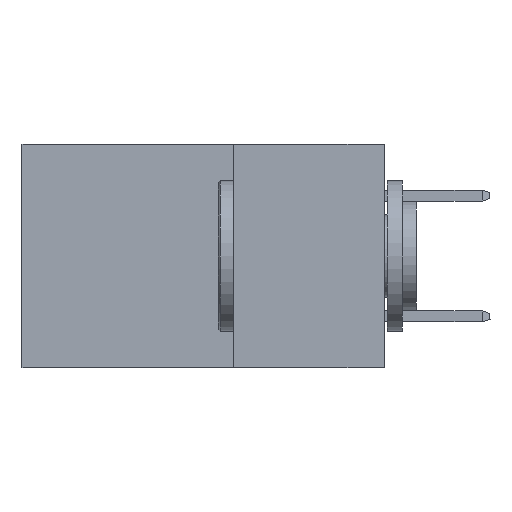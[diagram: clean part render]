
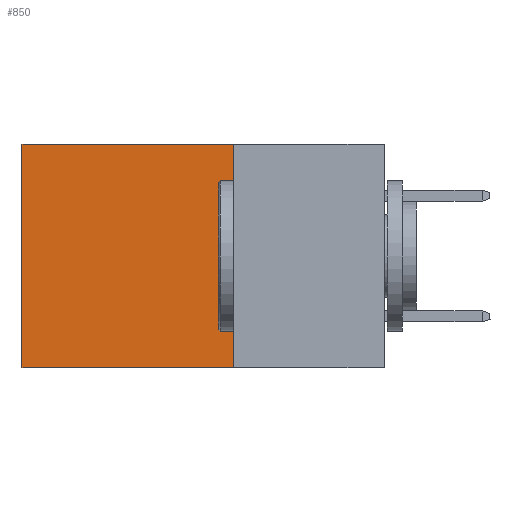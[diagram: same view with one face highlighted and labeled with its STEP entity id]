
A CAD part, left-side view. The second image highlights one B-rep face of the part: STEP entity #850.
In plain terms, the highlighted planar face has unit normal (-1, 0, 0).
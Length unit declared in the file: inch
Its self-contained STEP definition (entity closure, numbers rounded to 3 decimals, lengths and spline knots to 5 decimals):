
#69 = DIRECTION ( 'NONE',  ( 0., 0., -1. ) ) ;
#105 = CARTESIAN_POINT ( 'NONE',  ( 0.2615, 0.25, 0. ) ) ;
#148 = VECTOR ( 'NONE', #69, 39.37008 ) ;
#746 = DIRECTION ( 'NONE',  ( 0., 1., 0. ) ) ;
#850 = ADVANCED_FACE ( 'NONE', ( #4565 ), #6537, .F. ) ;
#1042 = CARTESIAN_POINT ( 'NONE',  ( 0.2615, 0.25, 0. ) ) ;
#1070 = VERTEX_POINT ( 'NONE', #1042 ) ;
#1103 = VERTEX_POINT ( 'NONE', #5256 ) ;
#1482 = EDGE_CURVE ( 'NONE', #1070, #8542, #1595, .T. ) ;
#1595 = LINE ( 'NONE', #105, #8017 ) ;
#1862 = ORIENTED_EDGE ( 'NONE', *, *, #10503, .F. ) ;
#3013 = ORIENTED_EDGE ( 'NONE', *, *, #5291, .F. ) ;
#3477 = AXIS2_PLACEMENT_3D ( 'NONE', #4935, #9805, #7328 ) ;
#3696 = VERTEX_POINT ( 'NONE', #4940 ) ;
#4012 = CARTESIAN_POINT ( 'NONE',  ( 0.2615, 0.6, -0.37 ) ) ;
#4186 = LINE ( 'NONE', #8465, #148 ) ;
#4358 = DIRECTION ( 'NONE',  ( 0., 1., 0. ) ) ;
#4565 = FACE_OUTER_BOUND ( 'NONE', #5736, .T. ) ;
#4592 = ORIENTED_EDGE ( 'NONE', *, *, #10613, .T. ) ;
#4624 = VECTOR ( 'NONE', #746, 39.37008 ) ;
#4889 = VECTOR ( 'NONE', #7412, 39.37008 ) ;
#4935 = CARTESIAN_POINT ( 'NONE',  ( 0.2615, 0.25, -0.37 ) ) ;
#4940 = CARTESIAN_POINT ( 'NONE',  ( 0.2615, 0.25, -0.37 ) ) ;
#5256 = CARTESIAN_POINT ( 'NONE',  ( 0.2615, 0.6, -0.37 ) ) ;
#5291 = EDGE_CURVE ( 'NONE', #1070, #3696, #4186, .T. ) ;
#5672 = LINE ( 'NONE', #4012, #4889 ) ;
#5736 = EDGE_LOOP ( 'NONE', ( #4592, #1862, #3013, #10686 ) ) ;
#6537 = PLANE ( 'NONE',  #3477 ) ;
#7328 = DIRECTION ( 'NONE',  ( 0., 0., -1. ) ) ;
#7412 = DIRECTION ( 'NONE',  ( 0., 0., -1. ) ) ;
#7909 = CARTESIAN_POINT ( 'NONE',  ( 0.2615, 0.6, 0. ) ) ;
#8017 = VECTOR ( 'NONE', #4358, 39.37008 ) ;
#8465 = CARTESIAN_POINT ( 'NONE',  ( 0.2615, 0.25, -0.37 ) ) ;
#8542 = VERTEX_POINT ( 'NONE', #7909 ) ;
#9805 = DIRECTION ( 'NONE',  ( 1., 0., 0. ) ) ;
#9971 = CARTESIAN_POINT ( 'NONE',  ( 0.2615, 0.25, -0.37 ) ) ;
#10503 = EDGE_CURVE ( 'NONE', #3696, #1103, #10649, .T. ) ;
#10613 = EDGE_CURVE ( 'NONE', #8542, #1103, #5672, .T. ) ;
#10649 = LINE ( 'NONE', #9971, #4624 ) ;
#10686 = ORIENTED_EDGE ( 'NONE', *, *, #1482, .T. ) ;
